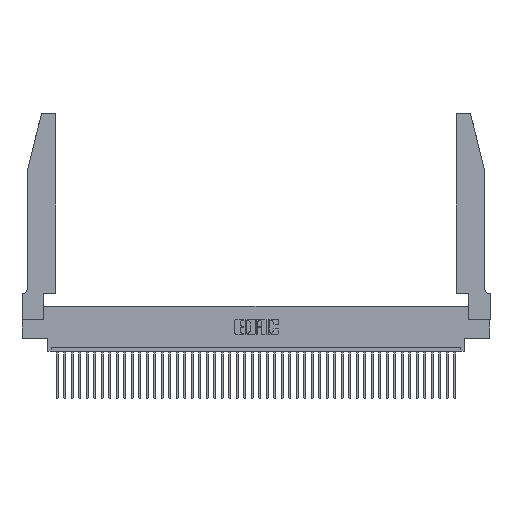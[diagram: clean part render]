
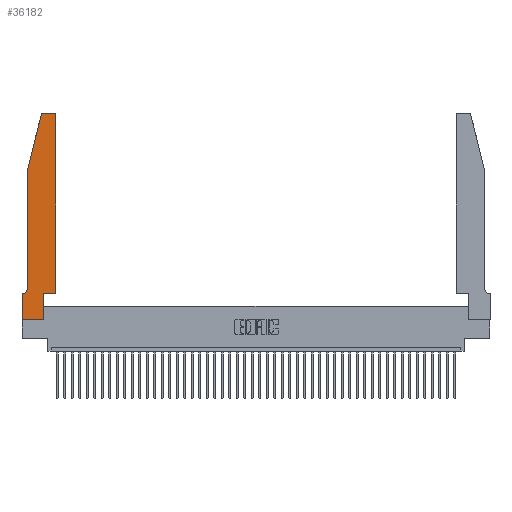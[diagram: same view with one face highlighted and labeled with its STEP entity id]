
A CAD part, top view. The second image highlights one B-rep face of the part: STEP entity #36182.
In plain terms, the highlighted planar face has unit normal (0, 0, 1).
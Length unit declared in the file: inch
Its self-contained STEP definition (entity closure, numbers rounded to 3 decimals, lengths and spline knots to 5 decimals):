
#154 = DIRECTION ( 'NONE',  ( 0., 0., 1. ) ) ;
#276 = CARTESIAN_POINT ( 'NONE',  ( 0.4205, 2.72, 0.37 ) ) ;
#371 = CIRCLE ( 'NONE', #20726, 0.07 ) ;
#493 = CARTESIAN_POINT ( 'NONE',  ( 0.284, 2.72, 0.37 ) ) ;
#885 = DIRECTION ( 'NONE',  ( 0., -1., 0. ) ) ;
#1483 = LINE ( 'NONE', #14032, #21155 ) ;
#1487 = CARTESIAN_POINT ( 'NONE',  ( 0.2865, 0.35, 0.37 ) ) ;
#1665 = CARTESIAN_POINT ( 'NONE',  ( 0., 0.35, 0.37 ) ) ;
#1706 = DIRECTION ( 'NONE',  ( 1., 0., 0. ) ) ;
#1749 = ORIENTED_EDGE ( 'NONE', *, *, #8099, .T. ) ;
#2458 = EDGE_CURVE ( 'NONE', #29646, #24973, #27231, .T. ) ;
#2666 = CARTESIAN_POINT ( 'NONE',  ( 0.4505, 0.35, 0.37 ) ) ;
#5137 = CARTESIAN_POINT ( 'NONE',  ( 0.2605, 2.75, 0.37 ) ) ;
#8099 = EDGE_CURVE ( 'NONE', #30441, #20085, #28358, .T. ) ;
#8160 = CARTESIAN_POINT ( 'NONE',  ( 0., 0., 0.37 ) ) ;
#8269 = VERTEX_POINT ( 'NONE', #33307 ) ;
#8376 = DIRECTION ( 'NONE',  ( 1., 0., 0. ) ) ;
#8504 = DIRECTION ( 'NONE',  ( 0., 0., 1. ) ) ;
#8505 = DIRECTION ( 'NONE',  ( -0.239, -0.971, 0. ) ) ;
#8642 = VERTEX_POINT ( 'NONE', #24798 ) ;
#8797 = VERTEX_POINT ( 'NONE', #35417 ) ;
#9063 = ORIENTED_EDGE ( 'NONE', *, *, #39076, .T. ) ;
#9143 = ORIENTED_EDGE ( 'NONE', *, *, #32810, .T. ) ;
#9249 = CARTESIAN_POINT ( 'NONE',  ( 0.4505, 2.72, 0.37 ) ) ;
#9413 = DIRECTION ( 'NONE',  ( -1., 0., 0. ) ) ;
#10376 = EDGE_CURVE ( 'NONE', #23092, #29646, #12197, .T. ) ;
#11651 = AXIS2_PLACEMENT_3D ( 'NONE', #1665, #8504, #22454 ) ;
#11939 = VECTOR ( 'NONE', #17637, 39.37008 ) ;
#12197 = CIRCLE ( 'NONE', #24636, 0.03 ) ;
#13045 = LINE ( 'NONE', #14608, #11939 ) ;
#13234 = ORIENTED_EDGE ( 'NONE', *, *, #20186, .T. ) ;
#13993 = EDGE_CURVE ( 'NONE', #8269, #38327, #36786, .T. ) ;
#14032 = CARTESIAN_POINT ( 'NONE',  ( 0.0755, 2., 0.37 ) ) ;
#14412 = CIRCLE ( 'NONE', #19634, 0.03 ) ;
#14608 = CARTESIAN_POINT ( 'NONE',  ( 0.0755, 0.35, 0.37 ) ) ;
#14865 = EDGE_CURVE ( 'NONE', #20085, #8642, #14412, .T. ) ;
#15118 = EDGE_CURVE ( 'NONE', #8642, #23092, #40379, .T. ) ;
#15227 = DIRECTION ( 'NONE',  ( 0., 0., 1. ) ) ;
#15565 = VECTOR ( 'NONE', #21661, 39.37008 ) ;
#15585 = CARTESIAN_POINT ( 'NONE',  ( 0.4505, 0.35, 0.37 ) ) ;
#16121 = CARTESIAN_POINT ( 'NONE',  ( 0.0055, 0.42, 0.37 ) ) ;
#16494 = VERTEX_POINT ( 'NONE', #19455 ) ;
#16572 = ORIENTED_EDGE ( 'NONE', *, *, #15118, .T. ) ;
#17229 = VECTOR ( 'NONE', #1706, 39.37008 ) ;
#17637 = DIRECTION ( 'NONE',  ( -1., 0., 0. ) ) ;
#18196 = VECTOR ( 'NONE', #8505, 39.37008 ) ;
#18317 = ORIENTED_EDGE ( 'NONE', *, *, #13993, .T. ) ;
#18395 = DIRECTION ( 'NONE',  ( 0., 1., 0. ) ) ;
#18612 = ORIENTED_EDGE ( 'NONE', *, *, #2458, .T. ) ;
#19455 = CARTESIAN_POINT ( 'NONE',  ( 0., 0., 0.37 ) ) ;
#19634 = AXIS2_PLACEMENT_3D ( 'NONE', #276, #154, #41359 ) ;
#20001 = ORIENTED_EDGE ( 'NONE', *, *, #37763, .T. ) ;
#20085 = VERTEX_POINT ( 'NONE', #9249 ) ;
#20186 = EDGE_CURVE ( 'NONE', #24973, #8797, #1483, .T. ) ;
#20726 = AXIS2_PLACEMENT_3D ( 'NONE', #16121, #29910, #9413 ) ;
#20839 = EDGE_CURVE ( 'NONE', #8797, #37386, #371, .T. ) ;
#20865 = LINE ( 'NONE', #22036, #17229 ) ;
#21155 = VECTOR ( 'NONE', #23954, 39.37008 ) ;
#21219 = EDGE_CURVE ( 'NONE', #38327, #30441, #30136, .T. ) ;
#21250 = VECTOR ( 'NONE', #32445, 39.37008 ) ;
#21661 = DIRECTION ( 'NONE',  ( 0., 1., 0. ) ) ;
#21992 = PLANE ( 'NONE',  #11651 ) ;
#22036 = CARTESIAN_POINT ( 'NONE',  ( 0., 0., 0.37 ) ) ;
#22454 = DIRECTION ( 'NONE',  ( 1., 0., 0. ) ) ;
#22592 = VECTOR ( 'NONE', #885, 39.37008 ) ;
#22852 = DIRECTION ( 'NONE',  ( 1., 0., 0. ) ) ;
#23092 = VERTEX_POINT ( 'NONE', #40231 ) ;
#23954 = DIRECTION ( 'NONE',  ( 0., -1., 0. ) ) ;
#24055 = CARTESIAN_POINT ( 'NONE',  ( 0.25487, 2.72718, 0.37 ) ) ;
#24407 = ORIENTED_EDGE ( 'NONE', *, *, #10376, .T. ) ;
#24467 = CARTESIAN_POINT ( 'NONE',  ( 0.2865, 0.35, 0.37 ) ) ;
#24636 = AXIS2_PLACEMENT_3D ( 'NONE', #493, #15227, #8376 ) ;
#24798 = CARTESIAN_POINT ( 'NONE',  ( 0.4205, 2.75, 0.37 ) ) ;
#24861 = CARTESIAN_POINT ( 'NONE',  ( 0.0055, 0.35, 0.37 ) ) ;
#24973 = VERTEX_POINT ( 'NONE', #43136 ) ;
#25321 = ORIENTED_EDGE ( 'NONE', *, *, #14865, .T. ) ;
#25888 = CARTESIAN_POINT ( 'NONE',  ( 0.0755, 2., 0.37 ) ) ;
#26084 = ORIENTED_EDGE ( 'NONE', *, *, #20839, .T. ) ;
#27231 = LINE ( 'NONE', #25888, #18196 ) ;
#27525 = FACE_OUTER_BOUND ( 'NONE', #39394, .T. ) ;
#28339 = CARTESIAN_POINT ( 'NONE',  ( 0., 0.35, 0.37 ) ) ;
#28358 = LINE ( 'NONE', #15585, #28880 ) ;
#28880 = VECTOR ( 'NONE', #18395, 39.37008 ) ;
#29646 = VERTEX_POINT ( 'NONE', #24055 ) ;
#29910 = DIRECTION ( 'NONE',  ( 0., 0., -1. ) ) ;
#30136 = LINE ( 'NONE', #2666, #38528 ) ;
#30441 = VERTEX_POINT ( 'NONE', #35335 ) ;
#32097 = VERTEX_POINT ( 'NONE', #28339 ) ;
#32445 = DIRECTION ( 'NONE',  ( -1., 0., 0. ) ) ;
#32810 = EDGE_CURVE ( 'NONE', #16494, #8269, #20865, .T. ) ;
#33307 = CARTESIAN_POINT ( 'NONE',  ( 0.2865, 0., 0.37 ) ) ;
#35335 = CARTESIAN_POINT ( 'NONE',  ( 0.4505, 0.35, 0.37 ) ) ;
#35417 = CARTESIAN_POINT ( 'NONE',  ( 0.0755, 0.42, 0.37 ) ) ;
#36182 = ADVANCED_FACE ( 'NONE', ( #27525 ), #21992, .T. ) ;
#36369 = LINE ( 'NONE', #8160, #22592 ) ;
#36786 = LINE ( 'NONE', #1487, #15565 ) ;
#37386 = VERTEX_POINT ( 'NONE', #24861 ) ;
#37763 = EDGE_CURVE ( 'NONE', #32097, #16494, #36369, .T. ) ;
#38327 = VERTEX_POINT ( 'NONE', #24467 ) ;
#38528 = VECTOR ( 'NONE', #22852, 39.37008 ) ;
#39076 = EDGE_CURVE ( 'NONE', #37386, #32097, #13045, .T. ) ;
#39394 = EDGE_LOOP ( 'NONE', ( #16572, #24407, #18612, #13234, #26084, #9063, #20001, #9143, #18317, #40634, #1749, #25321 ) ) ;
#40231 = CARTESIAN_POINT ( 'NONE',  ( 0.284, 2.75, 0.37 ) ) ;
#40379 = LINE ( 'NONE', #5137, #21250 ) ;
#40634 = ORIENTED_EDGE ( 'NONE', *, *, #21219, .T. ) ;
#41359 = DIRECTION ( 'NONE',  ( 1., 0., 0. ) ) ;
#43136 = CARTESIAN_POINT ( 'NONE',  ( 0.0755, 2., 0.37 ) ) ;
